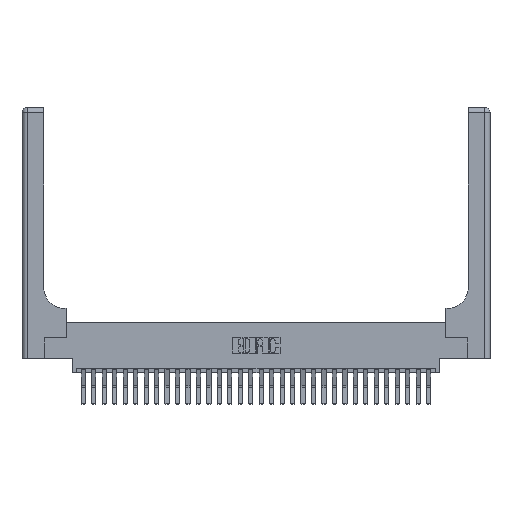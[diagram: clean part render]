
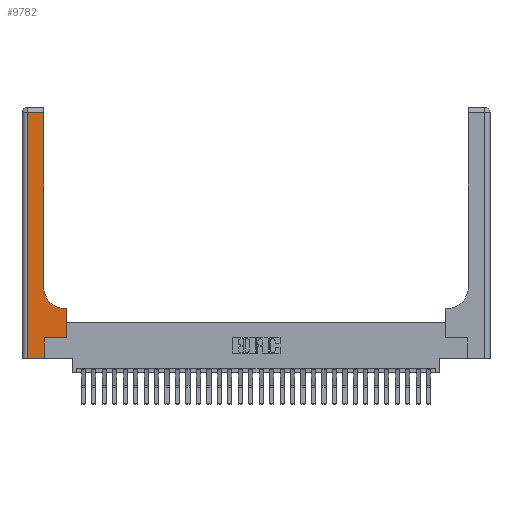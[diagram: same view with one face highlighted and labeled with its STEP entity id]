
A CAD part, top view. The second image highlights one B-rep face of the part: STEP entity #9782.
In plain terms, the highlighted planar face has unit normal (0, 0, 1).
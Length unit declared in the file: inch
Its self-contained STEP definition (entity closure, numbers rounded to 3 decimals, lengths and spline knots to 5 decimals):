
#58 = VECTOR ( 'NONE', #18930, 39.37008 ) ;
#109 = EDGE_CURVE ( 'NONE', #26146, #6497, #8064, .T. ) ;
#160 = CARTESIAN_POINT ( 'NONE',  ( 0.51, 0.6, 0.37 ) ) ;
#963 = CARTESIAN_POINT ( 'NONE',  ( 0.26, 3., 0.37 ) ) ;
#1727 = ORIENTED_EDGE ( 'NONE', *, *, #15332, .T. ) ;
#1955 = CARTESIAN_POINT ( 'NONE',  ( 0.06, 3., 0.37 ) ) ;
#2011 = CARTESIAN_POINT ( 'NONE',  ( 0.265, 0.25, 0.37 ) ) ;
#2392 = CARTESIAN_POINT ( 'NONE',  ( 0., 2.94, 0.37 ) ) ;
#2490 = CARTESIAN_POINT ( 'NONE',  ( 0.51, 0.85, 0.37 ) ) ;
#3376 = AXIS2_PLACEMENT_3D ( 'NONE', #2490, #18006, #4716 ) ;
#3444 = CARTESIAN_POINT ( 'NONE',  ( 0.26, 0.6, 0.37 ) ) ;
#3555 = ORIENTED_EDGE ( 'NONE', *, *, #25584, .T. ) ;
#3849 = VERTEX_POINT ( 'NONE', #20445 ) ;
#4197 = DIRECTION ( 'NONE',  ( 0., -1., 0. ) ) ;
#4299 = VERTEX_POINT ( 'NONE', #2011 ) ;
#4391 = EDGE_CURVE ( 'NONE', #3849, #10885, #4727, .T. ) ;
#4537 = DIRECTION ( 'NONE',  ( -1., 0., 0. ) ) ;
#4716 = DIRECTION ( 'NONE',  ( 1., 0., 0. ) ) ;
#4727 = LINE ( 'NONE', #2392, #15120 ) ;
#4858 = VERTEX_POINT ( 'NONE', #12115 ) ;
#4978 = VECTOR ( 'NONE', #4197, 39.37008 ) ;
#5208 = VERTEX_POINT ( 'NONE', #20506 ) ;
#5267 = CARTESIAN_POINT ( 'NONE',  ( 0.528, 0.25, 0.37 ) ) ;
#5887 = CARTESIAN_POINT ( 'NONE',  ( 0.265, 0., 0.37 ) ) ;
#6497 = VERTEX_POINT ( 'NONE', #11933 ) ;
#6640 = CARTESIAN_POINT ( 'NONE',  ( 0.265, 0.25, 0.37 ) ) ;
#6678 = DIRECTION ( 'NONE',  ( 0., 0., -1. ) ) ;
#6709 = AXIS2_PLACEMENT_3D ( 'NONE', #26544, #6678, #22178 ) ;
#6746 = VECTOR ( 'NONE', #19942, 39.37008 ) ;
#7354 = VECTOR ( 'NONE', #10937, 39.37008 ) ;
#8064 = LINE ( 'NONE', #26394, #7354 ) ;
#8458 = VERTEX_POINT ( 'NONE', #160 ) ;
#9782 = ADVANCED_FACE ( 'NONE', ( #14777 ), #19981, .F. ) ;
#10341 = EDGE_CURVE ( 'NONE', #4299, #4858, #24447, .T. ) ;
#10845 = ORIENTED_EDGE ( 'NONE', *, *, #24970, .T. ) ;
#10885 = VERTEX_POINT ( 'NONE', #21743 ) ;
#10937 = DIRECTION ( 'NONE',  ( 1., 0., 0. ) ) ;
#11543 = ORIENTED_EDGE ( 'NONE', *, *, #24246, .T. ) ;
#11933 = CARTESIAN_POINT ( 'NONE',  ( 0.265, 0., 0.37 ) ) ;
#12115 = CARTESIAN_POINT ( 'NONE',  ( 0.528, 0.25, 0.37 ) ) ;
#13214 = ORIENTED_EDGE ( 'NONE', *, *, #10341, .T. ) ;
#13723 = EDGE_CURVE ( 'NONE', #17543, #3849, #28578, .T. ) ;
#14662 = VECTOR ( 'NONE', #19089, 39.37008 ) ;
#14777 = FACE_OUTER_BOUND ( 'NONE', #19519, .T. ) ;
#15120 = VECTOR ( 'NONE', #4537, 39.37008 ) ;
#15332 = EDGE_CURVE ( 'NONE', #10885, #26146, #22657, .T. ) ;
#15924 = EDGE_CURVE ( 'NONE', #6497, #4299, #20550, .T. ) ;
#17543 = VERTEX_POINT ( 'NONE', #20557 ) ;
#18006 = DIRECTION ( 'NONE',  ( 0., 0., -1. ) ) ;
#18169 = CIRCLE ( 'NONE', #3376, 0.25 ) ;
#18579 = DIRECTION ( 'NONE',  ( 0., 1., 0. ) ) ;
#18721 = DIRECTION ( 'NONE',  ( 0., 1., 0. ) ) ;
#18728 = ORIENTED_EDGE ( 'NONE', *, *, #13723, .T. ) ;
#18789 = VECTOR ( 'NONE', #18579, 39.37008 ) ;
#18930 = DIRECTION ( 'NONE',  ( -1., 0., 0. ) ) ;
#19089 = DIRECTION ( 'NONE',  ( 0., 1., 0. ) ) ;
#19519 = EDGE_LOOP ( 'NONE', ( #18728, #25293, #1727, #21522, #22908, #13214, #3555, #10845, #11543 ) ) ;
#19942 = DIRECTION ( 'NONE',  ( 1., 0., 0. ) ) ;
#19981 = PLANE ( 'NONE',  #6709 ) ;
#20445 = CARTESIAN_POINT ( 'NONE',  ( 0.26, 2.94, 0.37 ) ) ;
#20506 = CARTESIAN_POINT ( 'NONE',  ( 0.528, 0.6, 0.37 ) ) ;
#20550 = LINE ( 'NONE', #5887, #14662 ) ;
#20557 = CARTESIAN_POINT ( 'NONE',  ( 0.26, 0.85, 0.37 ) ) ;
#21522 = ORIENTED_EDGE ( 'NONE', *, *, #109, .T. ) ;
#21743 = CARTESIAN_POINT ( 'NONE',  ( 0.06, 2.94, 0.37 ) ) ;
#22178 = DIRECTION ( 'NONE',  ( -1., 0., 0. ) ) ;
#22657 = LINE ( 'NONE', #1955, #4978 ) ;
#22779 = CARTESIAN_POINT ( 'NONE',  ( 0.06, 0., 0.37 ) ) ;
#22908 = ORIENTED_EDGE ( 'NONE', *, *, #15924, .T. ) ;
#22956 = LINE ( 'NONE', #3444, #58 ) ;
#24246 = EDGE_CURVE ( 'NONE', #8458, #17543, #18169, .T. ) ;
#24447 = LINE ( 'NONE', #6640, #6746 ) ;
#24970 = EDGE_CURVE ( 'NONE', #5208, #8458, #22956, .T. ) ;
#25293 = ORIENTED_EDGE ( 'NONE', *, *, #4391, .T. ) ;
#25352 = LINE ( 'NONE', #5267, #18789 ) ;
#25584 = EDGE_CURVE ( 'NONE', #4858, #5208, #25352, .T. ) ;
#26146 = VERTEX_POINT ( 'NONE', #22779 ) ;
#26394 = CARTESIAN_POINT ( 'NONE',  ( 0., 0., 0.37 ) ) ;
#26544 = CARTESIAN_POINT ( 'NONE',  ( 0., 3., 0.37 ) ) ;
#27885 = VECTOR ( 'NONE', #18721, 39.37008 ) ;
#28578 = LINE ( 'NONE', #963, #27885 ) ;
